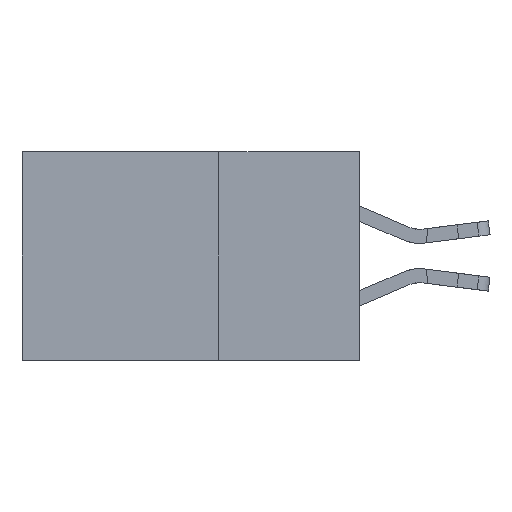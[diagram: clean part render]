
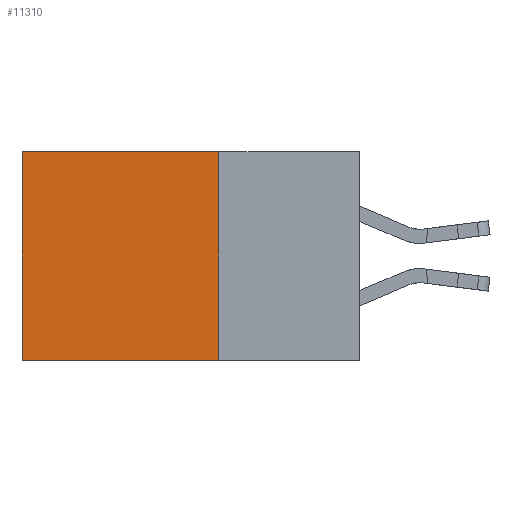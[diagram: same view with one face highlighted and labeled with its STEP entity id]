
A CAD part, left-side view. The second image highlights one B-rep face of the part: STEP entity #11310.
In plain terms, the highlighted planar face has unit normal (-1, 0, 0).
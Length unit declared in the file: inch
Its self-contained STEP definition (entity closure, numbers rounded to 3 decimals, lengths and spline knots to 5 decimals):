
#90 = EDGE_CURVE ( 'NONE', #16167, #3892, #7362, .T. ) ;
#144 = AXIS2_PLACEMENT_3D ( 'NONE', #4193, #16095, #2964 ) ;
#451 = VECTOR ( 'NONE', #3006, 39.37008 ) ;
#755 = ORIENTED_EDGE ( 'NONE', *, *, #13249, .F. ) ;
#1028 = EDGE_LOOP ( 'NONE', ( #9777, #755, #14573, #4838 ) ) ;
#1435 = CARTESIAN_POINT ( 'NONE',  ( 0.2875, 0.25, -0.37 ) ) ;
#1498 = VERTEX_POINT ( 'NONE', #12632 ) ;
#1510 = PLANE ( 'NONE',  #144 ) ;
#1534 = CARTESIAN_POINT ( 'NONE',  ( 0.2875, 0.6, 0. ) ) ;
#2964 = DIRECTION ( 'NONE',  ( 0., 0., -1. ) ) ;
#3006 = DIRECTION ( 'NONE',  ( 0., 1., 0. ) ) ;
#3892 = VERTEX_POINT ( 'NONE', #1435 ) ;
#4193 = CARTESIAN_POINT ( 'NONE',  ( 0.2875, 0.25, 0. ) ) ;
#4278 = VECTOR ( 'NONE', #14053, 39.37008 ) ;
#4838 = ORIENTED_EDGE ( 'NONE', *, *, #9773, .T. ) ;
#5301 = CARTESIAN_POINT ( 'NONE',  ( 0.2875, 0.25, 0. ) ) ;
#7332 = CARTESIAN_POINT ( 'NONE',  ( 0.2875, 0.25, -0.37 ) ) ;
#7362 = LINE ( 'NONE', #15873, #4278 ) ;
#8663 = DIRECTION ( 'NONE',  ( 0., 1., 0. ) ) ;
#9360 = LINE ( 'NONE', #7332, #12194 ) ;
#9773 = EDGE_CURVE ( 'NONE', #16167, #10651, #11583, .T. ) ;
#9777 = ORIENTED_EDGE ( 'NONE', *, *, #14126, .T. ) ;
#10651 = VERTEX_POINT ( 'NONE', #1534 ) ;
#10963 = VECTOR ( 'NONE', #14388, 39.37008 ) ;
#11310 = ADVANCED_FACE ( 'NONE', ( #13074 ), #1510, .F. ) ;
#11583 = LINE ( 'NONE', #13179, #451 ) ;
#12194 = VECTOR ( 'NONE', #8663, 39.37008 ) ;
#12632 = CARTESIAN_POINT ( 'NONE',  ( 0.2875, 0.6, -0.37 ) ) ;
#13074 = FACE_OUTER_BOUND ( 'NONE', #1028, .T. ) ;
#13179 = CARTESIAN_POINT ( 'NONE',  ( 0.2875, 0.25, 0. ) ) ;
#13249 = EDGE_CURVE ( 'NONE', #3892, #1498, #9360, .T. ) ;
#14053 = DIRECTION ( 'NONE',  ( 0., 0., -1. ) ) ;
#14126 = EDGE_CURVE ( 'NONE', #10651, #1498, #14445, .T. ) ;
#14388 = DIRECTION ( 'NONE',  ( 0., 0., -1. ) ) ;
#14445 = LINE ( 'NONE', #16976, #10963 ) ;
#14573 = ORIENTED_EDGE ( 'NONE', *, *, #90, .F. ) ;
#15873 = CARTESIAN_POINT ( 'NONE',  ( 0.2875, 0.25, 0. ) ) ;
#16095 = DIRECTION ( 'NONE',  ( 1., 0., 0. ) ) ;
#16167 = VERTEX_POINT ( 'NONE', #5301 ) ;
#16976 = CARTESIAN_POINT ( 'NONE',  ( 0.2875, 0.6, 0. ) ) ;
